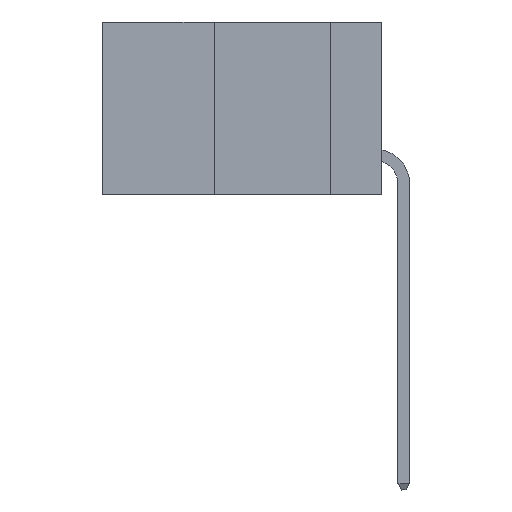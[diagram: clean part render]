
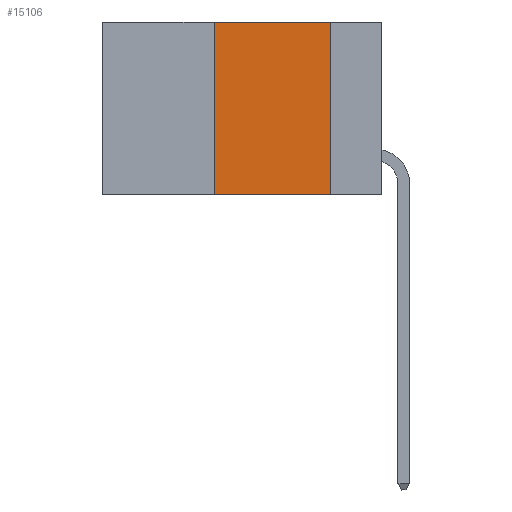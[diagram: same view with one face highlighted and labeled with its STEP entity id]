
A CAD part, left-side view. The second image highlights one B-rep face of the part: STEP entity #15106.
In plain terms, the highlighted planar face has unit normal (-1, 0, 0).
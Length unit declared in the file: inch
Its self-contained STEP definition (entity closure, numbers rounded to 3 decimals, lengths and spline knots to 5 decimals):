
#391 = ORIENTED_EDGE ( 'NONE', *, *, #43501, .F. ) ;
#877 = DIRECTION ( 'NONE',  ( 0., -1., 0. ) ) ;
#1263 = VERTEX_POINT ( 'NONE', #39999 ) ;
#1408 = LINE ( 'NONE', #25859, #35951 ) ;
#3896 = LINE ( 'NONE', #4654, #23947 ) ;
#4654 = CARTESIAN_POINT ( 'NONE',  ( 0., 0.6, -0.37 ) ) ;
#6377 = LINE ( 'NONE', #22564, #10206 ) ;
#6553 = CARTESIAN_POINT ( 'NONE',  ( 0., 0.11, -0.37 ) ) ;
#9494 = AXIS2_PLACEMENT_3D ( 'NONE', #24000, #20753, #41967 ) ;
#10206 = VECTOR ( 'NONE', #40692, 39.37008 ) ;
#12814 = LINE ( 'NONE', #21830, #41262 ) ;
#13372 = ORIENTED_EDGE ( 'NONE', *, *, #19214, .T. ) ;
#13720 = FACE_OUTER_BOUND ( 'NONE', #32956, .T. ) ;
#15106 = ADVANCED_FACE ( 'NONE', ( #13720 ), #34511, .F. ) ;
#17927 = ORIENTED_EDGE ( 'NONE', *, *, #32445, .F. ) ;
#19214 = EDGE_CURVE ( 'NONE', #29820, #19278, #3896, .T. ) ;
#19227 = DIRECTION ( 'NONE',  ( 0., 0., 1. ) ) ;
#19278 = VERTEX_POINT ( 'NONE', #6553 ) ;
#20753 = DIRECTION ( 'NONE',  ( 1., 0., 0. ) ) ;
#21432 = CARTESIAN_POINT ( 'NONE',  ( 0., 0.36, 0. ) ) ;
#21830 = CARTESIAN_POINT ( 'NONE',  ( 0., 0.11, 0. ) ) ;
#22564 = CARTESIAN_POINT ( 'NONE',  ( 0., 0.6, 0. ) ) ;
#23947 = VECTOR ( 'NONE', #877, 39.37008 ) ;
#24000 = CARTESIAN_POINT ( 'NONE',  ( 0., 0.6, 0. ) ) ;
#25859 = CARTESIAN_POINT ( 'NONE',  ( 0., 0.36, 0. ) ) ;
#29134 = DIRECTION ( 'NONE',  ( 0., 0., -1. ) ) ;
#29554 = ORIENTED_EDGE ( 'NONE', *, *, #31376, .F. ) ;
#29820 = VERTEX_POINT ( 'NONE', #31049 ) ;
#31049 = CARTESIAN_POINT ( 'NONE',  ( 0., 0.36, -0.37 ) ) ;
#31376 = EDGE_CURVE ( 'NONE', #29820, #40273, #1408, .T. ) ;
#32445 = EDGE_CURVE ( 'NONE', #40273, #1263, #6377, .T. ) ;
#32956 = EDGE_LOOP ( 'NONE', ( #391, #17927, #29554, #13372 ) ) ;
#34511 = PLANE ( 'NONE',  #9494 ) ;
#35951 = VECTOR ( 'NONE', #19227, 39.37008 ) ;
#39999 = CARTESIAN_POINT ( 'NONE',  ( 0., 0.11, 0. ) ) ;
#40273 = VERTEX_POINT ( 'NONE', #21432 ) ;
#40692 = DIRECTION ( 'NONE',  ( 0., -1., 0. ) ) ;
#41262 = VECTOR ( 'NONE', #29134, 39.37008 ) ;
#41967 = DIRECTION ( 'NONE',  ( 0., 0., -1. ) ) ;
#43501 = EDGE_CURVE ( 'NONE', #1263, #19278, #12814, .T. ) ;
